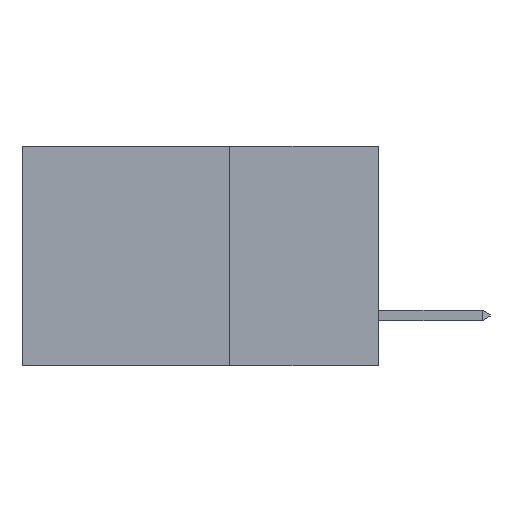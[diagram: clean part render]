
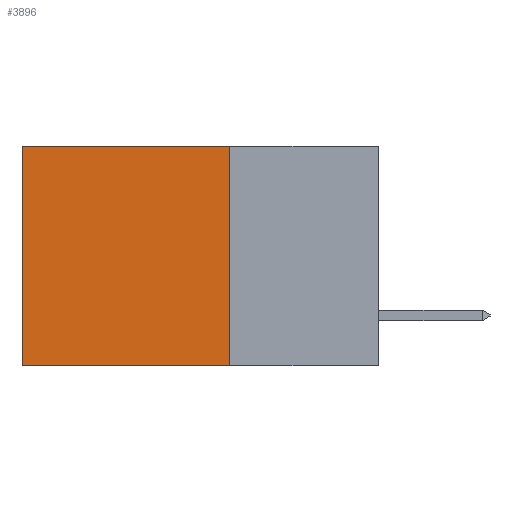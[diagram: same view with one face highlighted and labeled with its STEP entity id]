
A CAD part, left-side view. The second image highlights one B-rep face of the part: STEP entity #3896.
In plain terms, the highlighted planar face has unit normal (-1, 0, 0).
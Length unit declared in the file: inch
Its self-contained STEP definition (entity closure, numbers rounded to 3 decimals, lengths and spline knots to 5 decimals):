
#378 = VERTEX_POINT ( 'NONE', #8671 ) ;
#412 = EDGE_CURVE ( 'NONE', #7108, #378, #1870, .T. ) ;
#862 = CARTESIAN_POINT ( 'NONE',  ( 0.298, 0.6, -0.37 ) ) ;
#954 = DIRECTION ( 'NONE',  ( 0., 0., -1. ) ) ;
#1526 = CARTESIAN_POINT ( 'NONE',  ( 0.298, 0.25, 0. ) ) ;
#1742 = LINE ( 'NONE', #5003, #10193 ) ;
#1759 = ORIENTED_EDGE ( 'NONE', *, *, #412, .T. ) ;
#1845 = EDGE_LOOP ( 'NONE', ( #9517, #11138, #10311, #1759 ) ) ;
#1870 = LINE ( 'NONE', #9703, #7618 ) ;
#2608 = FACE_OUTER_BOUND ( 'NONE', #1845, .T. ) ;
#3723 = EDGE_CURVE ( 'NONE', #6132, #6576, #1742, .T. ) ;
#3807 = CARTESIAN_POINT ( 'NONE',  ( 0.298, 0.25, -0.37 ) ) ;
#3896 = ADVANCED_FACE ( 'NONE', ( #2608 ), #6903, .F. ) ;
#4095 = VECTOR ( 'NONE', #12397, 39.37008 ) ;
#4428 = LINE ( 'NONE', #6014, #11995 ) ;
#4870 = EDGE_CURVE ( 'NONE', #7108, #6132, #12600, .T. ) ;
#5003 = CARTESIAN_POINT ( 'NONE',  ( 0.298, 0.25, -0.37 ) ) ;
#6014 = CARTESIAN_POINT ( 'NONE',  ( 0.298, 0.6, 0. ) ) ;
#6132 = VERTEX_POINT ( 'NONE', #3807 ) ;
#6576 = VERTEX_POINT ( 'NONE', #862 ) ;
#6903 = PLANE ( 'NONE',  #12075 ) ;
#7108 = VERTEX_POINT ( 'NONE', #9076 ) ;
#7618 = VECTOR ( 'NONE', #9693, 39.37008 ) ;
#8671 = CARTESIAN_POINT ( 'NONE',  ( 0.298, 0.6, 0. ) ) ;
#9036 = DIRECTION ( 'NONE',  ( 1., 0., 0. ) ) ;
#9076 = CARTESIAN_POINT ( 'NONE',  ( 0.298, 0.25, 0. ) ) ;
#9517 = ORIENTED_EDGE ( 'NONE', *, *, #9797, .T. ) ;
#9693 = DIRECTION ( 'NONE',  ( 0., 1., 0. ) ) ;
#9703 = CARTESIAN_POINT ( 'NONE',  ( 0.298, 0.25, 0. ) ) ;
#9797 = EDGE_CURVE ( 'NONE', #378, #6576, #4428, .T. ) ;
#10193 = VECTOR ( 'NONE', #13391, 39.37008 ) ;
#10311 = ORIENTED_EDGE ( 'NONE', *, *, #4870, .F. ) ;
#11138 = ORIENTED_EDGE ( 'NONE', *, *, #3723, .F. ) ;
#11995 = VECTOR ( 'NONE', #13075, 39.37008 ) ;
#12075 = AXIS2_PLACEMENT_3D ( 'NONE', #1526, #9036, #954 ) ;
#12397 = DIRECTION ( 'NONE',  ( 0., 0., -1. ) ) ;
#12434 = CARTESIAN_POINT ( 'NONE',  ( 0.298, 0.25, 0. ) ) ;
#12600 = LINE ( 'NONE', #12434, #4095 ) ;
#13075 = DIRECTION ( 'NONE',  ( 0., 0., -1. ) ) ;
#13391 = DIRECTION ( 'NONE',  ( 0., 1., 0. ) ) ;
